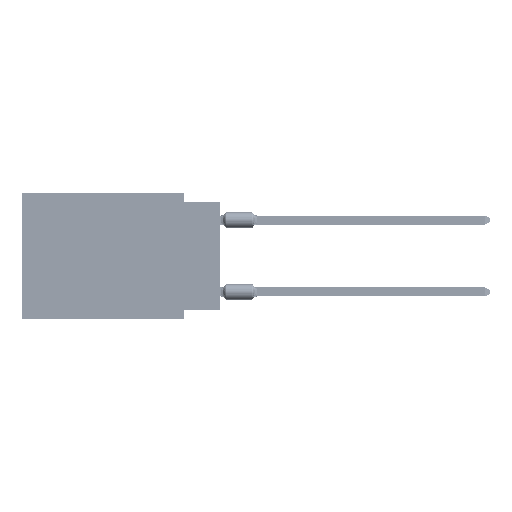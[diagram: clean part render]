
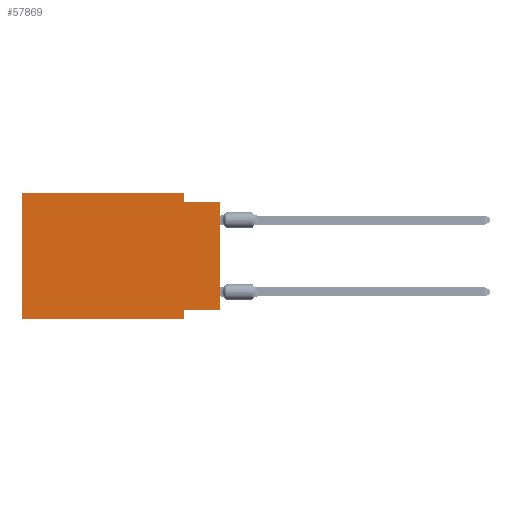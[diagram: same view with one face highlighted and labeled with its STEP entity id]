
A CAD part, left-side view. The second image highlights one B-rep face of the part: STEP entity #57869.
In plain terms, the highlighted planar face has unit normal (-1, 0, 0).
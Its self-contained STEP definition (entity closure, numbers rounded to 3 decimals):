
#659 = VERTEX_POINT ( 'NONE', #69891 ) ;
#4007 = VECTOR ( 'NONE', #49086, 1000. ) ;
#4368 = CARTESIAN_POINT ( 'NONE',  ( 0., 0., -0.635 ) ) ;
#5336 = ORIENTED_EDGE ( 'NONE', *, *, #62618, .F. ) ;
#10219 = EDGE_CURVE ( 'NONE', #48390, #659, #48934, .T. ) ;
#15056 = LINE ( 'NONE', #92947, #16390 ) ;
#16002 = CARTESIAN_POINT ( 'NONE',  ( 0., 13.97, -8.89 ) ) ;
#16390 = VECTOR ( 'NONE', #109083, 1000. ) ;
#16701 = VECTOR ( 'NONE', #112892, 1000. ) ;
#17558 = CARTESIAN_POINT ( 'NONE',  ( 0., 2.54, -0.635 ) ) ;
#18026 = VERTEX_POINT ( 'NONE', #17558 ) ;
#18367 = ORIENTED_EDGE ( 'NONE', *, *, #90433, .F. ) ;
#18928 = DIRECTION ( 'NONE',  ( 0., -1., 0. ) ) ;
#19489 = LINE ( 'NONE', #20032, #20874 ) ;
#20032 = CARTESIAN_POINT ( 'NONE',  ( 0., 2.54, -8.89 ) ) ;
#20267 = VECTOR ( 'NONE', #91812, 1000. ) ;
#20874 = VECTOR ( 'NONE', #29844, 1000. ) ;
#21335 = EDGE_LOOP ( 'NONE', ( #95479, #5336, #111555, #24958, #22657, #84655, #18367, #110691 ) ) ;
#21878 = DIRECTION ( 'NONE',  ( 1., 0., 0. ) ) ;
#22657 = ORIENTED_EDGE ( 'NONE', *, *, #10219, .F. ) ;
#23029 = CARTESIAN_POINT ( 'NONE',  ( 0., 2.54, 0. ) ) ;
#24461 = VERTEX_POINT ( 'NONE', #4368 ) ;
#24958 = ORIENTED_EDGE ( 'NONE', *, *, #88508, .F. ) ;
#27013 = CARTESIAN_POINT ( 'NONE',  ( 0., 0., -0.635 ) ) ;
#29694 = LINE ( 'NONE', #73524, #34808 ) ;
#29844 = DIRECTION ( 'NONE',  ( 0., 0., -1. ) ) ;
#29973 = PLANE ( 'NONE',  #102834 ) ;
#32683 = CARTESIAN_POINT ( 'NONE',  ( 0., 2.54, -8.89 ) ) ;
#34808 = VECTOR ( 'NONE', #109826, 1000. ) ;
#37352 = CARTESIAN_POINT ( 'NONE',  ( 0., 0., -8.255 ) ) ;
#38199 = VERTEX_POINT ( 'NONE', #32683 ) ;
#39762 = DIRECTION ( 'NONE',  ( 0., 0., -1. ) ) ;
#40311 = CARTESIAN_POINT ( 'NONE',  ( 0., 2.54, -8.255 ) ) ;
#48390 = VERTEX_POINT ( 'NONE', #54921 ) ;
#48934 = LINE ( 'NONE', #84104, #86579 ) ;
#49086 = DIRECTION ( 'NONE',  ( 0., -1., 0. ) ) ;
#54921 = CARTESIAN_POINT ( 'NONE',  ( 0., 13.97, -8.89 ) ) ;
#56515 = CARTESIAN_POINT ( 'NONE',  ( 0., 13.97, 0. ) ) ;
#56605 = LINE ( 'NONE', #83138, #4007 ) ;
#57869 = ADVANCED_FACE ( 'NONE', ( #84728 ), #29973, .F. ) ;
#58355 = LINE ( 'NONE', #67584, #20267 ) ;
#62618 = EDGE_CURVE ( 'NONE', #18026, #24461, #97912, .T. ) ;
#67584 = CARTESIAN_POINT ( 'NONE',  ( 0., 2.54, 0. ) ) ;
#67934 = LINE ( 'NONE', #16002, #16701 ) ;
#69398 = EDGE_CURVE ( 'NONE', #101502, #24461, #15056, .T. ) ;
#69891 = CARTESIAN_POINT ( 'NONE',  ( 0., 13.97, 0. ) ) ;
#70585 = EDGE_CURVE ( 'NONE', #94857, #18026, #58355, .T. ) ;
#73524 = CARTESIAN_POINT ( 'NONE',  ( 0., 0., -8.255 ) ) ;
#83138 = CARTESIAN_POINT ( 'NONE',  ( 0., 13.97, 0. ) ) ;
#84104 = CARTESIAN_POINT ( 'NONE',  ( 0., 13.97, 0. ) ) ;
#84655 = ORIENTED_EDGE ( 'NONE', *, *, #99147, .T. ) ;
#84728 = FACE_OUTER_BOUND ( 'NONE', #21335, .T. ) ;
#86579 = VECTOR ( 'NONE', #95011, 1000. ) ;
#88508 = EDGE_CURVE ( 'NONE', #659, #94857, #56605, .T. ) ;
#90433 = EDGE_CURVE ( 'NONE', #101188, #38199, #19489, .T. ) ;
#91812 = DIRECTION ( 'NONE',  ( 0., 0., -1. ) ) ;
#92947 = CARTESIAN_POINT ( 'NONE',  ( 0., 0., 0. ) ) ;
#94857 = VERTEX_POINT ( 'NONE', #23029 ) ;
#95011 = DIRECTION ( 'NONE',  ( 0., 0., 1. ) ) ;
#95479 = ORIENTED_EDGE ( 'NONE', *, *, #69398, .T. ) ;
#95582 = EDGE_CURVE ( 'NONE', #101502, #101188, #29694, .T. ) ;
#97912 = LINE ( 'NONE', #27013, #103327 ) ;
#99147 = EDGE_CURVE ( 'NONE', #48390, #38199, #67934, .T. ) ;
#101188 = VERTEX_POINT ( 'NONE', #40311 ) ;
#101502 = VERTEX_POINT ( 'NONE', #37352 ) ;
#102834 = AXIS2_PLACEMENT_3D ( 'NONE', #56515, #21878, #39762 ) ;
#103327 = VECTOR ( 'NONE', #18928, 1000. ) ;
#109083 = DIRECTION ( 'NONE',  ( 0., 0., 1. ) ) ;
#109826 = DIRECTION ( 'NONE',  ( 0., 1., 0. ) ) ;
#110691 = ORIENTED_EDGE ( 'NONE', *, *, #95582, .F. ) ;
#111555 = ORIENTED_EDGE ( 'NONE', *, *, #70585, .F. ) ;
#112892 = DIRECTION ( 'NONE',  ( 0., -1., 0. ) ) ;
